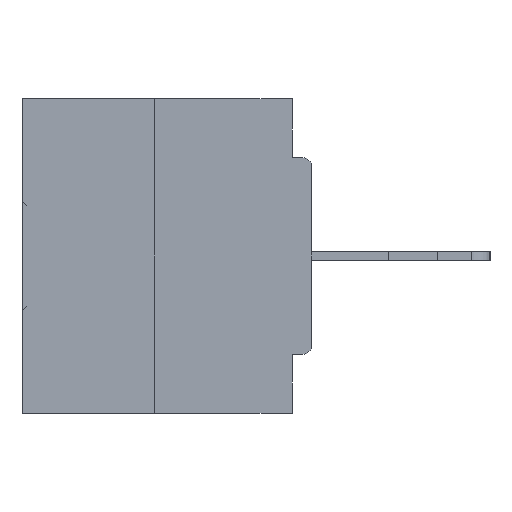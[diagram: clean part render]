
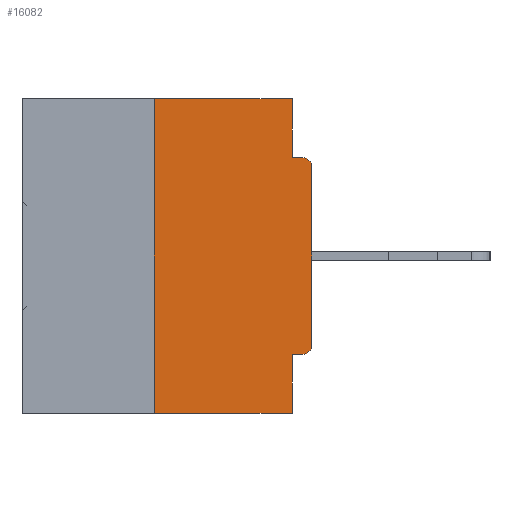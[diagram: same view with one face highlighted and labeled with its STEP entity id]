
A CAD part, left-side view. The second image highlights one B-rep face of the part: STEP entity #16082.
In plain terms, the highlighted planar face has unit normal (-1, 0, 0).
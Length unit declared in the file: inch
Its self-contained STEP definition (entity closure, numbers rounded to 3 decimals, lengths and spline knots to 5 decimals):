
#166 = CARTESIAN_POINT ( 'NONE',  ( 0., 0.031, -0.5 ) ) ;
#271 = DIRECTION ( 'NONE',  ( 0., 1., 0. ) ) ;
#1681 = DIRECTION ( 'NONE',  ( 0., 0., -1. ) ) ;
#2871 = CARTESIAN_POINT ( 'NONE',  ( 0., 0.031, -0.4065 ) ) ;
#3546 = DIRECTION ( 'NONE',  ( 0., 0., -1. ) ) ;
#4654 = CARTESIAN_POINT ( 'NONE',  ( 0., 0., -0.3915 ) ) ;
#5396 = CARTESIAN_POINT ( 'NONE',  ( 0., 0.015, -0.0935 ) ) ;
#5645 = CARTESIAN_POINT ( 'NONE',  ( 0., 0.25, -0.5 ) ) ;
#6188 = VERTEX_POINT ( 'NONE', #2871 ) ;
#6220 = CARTESIAN_POINT ( 'NONE',  ( 0., 0., -0.4065 ) ) ;
#7748 = ORIENTED_EDGE ( 'NONE', *, *, #12546, .T. ) ;
#8035 = CARTESIAN_POINT ( 'NONE',  ( 0., 0.031, -0.5 ) ) ;
#8219 = CARTESIAN_POINT ( 'NONE',  ( 0., 0., -0.0935 ) ) ;
#9398 = EDGE_LOOP ( 'NONE', ( #33979, #33507, #30368, #36195, #10634, #37885, #7748, #32452, #12230, #32280 ) ) ;
#9881 = CARTESIAN_POINT ( 'NONE',  ( 0., 0.031, 0. ) ) ;
#9919 = DIRECTION ( 'NONE',  ( -1., 0., 0. ) ) ;
#10634 = ORIENTED_EDGE ( 'NONE', *, *, #40237, .F. ) ;
#10736 = DIRECTION ( 'NONE',  ( -1., 0., 0. ) ) ;
#11632 = LINE ( 'NONE', #20674, #40457 ) ;
#12211 = EDGE_CURVE ( 'NONE', #38608, #39291, #38129, .T. ) ;
#12230 = ORIENTED_EDGE ( 'NONE', *, *, #25489, .F. ) ;
#12546 = EDGE_CURVE ( 'NONE', #26286, #21401, #11632, .T. ) ;
#14592 = FACE_OUTER_BOUND ( 'NONE', #9398, .T. ) ;
#15478 = EDGE_CURVE ( 'NONE', #6188, #39291, #18635, .T. ) ;
#16082 = ADVANCED_FACE ( 'NONE', ( #14592 ), #23435, .F. ) ;
#16759 = CARTESIAN_POINT ( 'NONE',  ( 0., 0.031, 0. ) ) ;
#17078 = CARTESIAN_POINT ( 'NONE',  ( 0., 0.015, -0.1085 ) ) ;
#17314 = LINE ( 'NONE', #26383, #34043 ) ;
#17432 = EDGE_CURVE ( 'NONE', #24392, #33461, #17314, .T. ) ;
#17445 = DIRECTION ( 'NONE',  ( 0., -1., 0. ) ) ;
#17661 = AXIS2_PLACEMENT_3D ( 'NONE', #28186, #9919, #3546 ) ;
#18257 = CARTESIAN_POINT ( 'NONE',  ( 0., 0.25, 0. ) ) ;
#18635 = LINE ( 'NONE', #166, #39279 ) ;
#18839 = DIRECTION ( 'NONE',  ( 0., 0., 1. ) ) ;
#19458 = CARTESIAN_POINT ( 'NONE',  ( 0., 0.46, -0.5 ) ) ;
#19953 = DIRECTION ( 'NONE',  ( 1., 0., 0. ) ) ;
#19972 = DIRECTION ( 'NONE',  ( 0., 0., -1. ) ) ;
#20674 = CARTESIAN_POINT ( 'NONE',  ( 0., 0., 0. ) ) ;
#21401 = VERTEX_POINT ( 'NONE', #38462 ) ;
#22126 = DIRECTION ( 'NONE',  ( 0., 0., -1. ) ) ;
#22452 = AXIS2_PLACEMENT_3D ( 'NONE', #17078, #10736, #19972 ) ;
#22699 = VECTOR ( 'NONE', #17445, 39.37008 ) ;
#23435 = PLANE ( 'NONE',  #26215 ) ;
#24304 = DIRECTION ( 'NONE',  ( 0., -1., 0. ) ) ;
#24392 = VERTEX_POINT ( 'NONE', #18257 ) ;
#24836 = VECTOR ( 'NONE', #18839, 39.37008 ) ;
#25211 = CARTESIAN_POINT ( 'NONE',  ( 0., 0.25, 0. ) ) ;
#25489 = EDGE_CURVE ( 'NONE', #27719, #30728, #40005, .T. ) ;
#26215 = AXIS2_PLACEMENT_3D ( 'NONE', #35519, #19953, #1681 ) ;
#26286 = VERTEX_POINT ( 'NONE', #4654 ) ;
#26383 = CARTESIAN_POINT ( 'NONE',  ( 0., 0.46, 0. ) ) ;
#26784 = CARTESIAN_POINT ( 'NONE',  ( 0., 0.015, -0.4065 ) ) ;
#27719 = VERTEX_POINT ( 'NONE', #34202 ) ;
#28186 = CARTESIAN_POINT ( 'NONE',  ( 0., 0.015, -0.3915 ) ) ;
#28669 = VECTOR ( 'NONE', #24304, 39.37008 ) ;
#30368 = ORIENTED_EDGE ( 'NONE', *, *, #12211, .T. ) ;
#30503 = DIRECTION ( 'NONE',  ( 0., 0., 1. ) ) ;
#30713 = VECTOR ( 'NONE', #38919, 39.37008 ) ;
#30728 = VERTEX_POINT ( 'NONE', #5396 ) ;
#31062 = LINE ( 'NONE', #6220, #37327 ) ;
#31638 = VERTEX_POINT ( 'NONE', #26784 ) ;
#32280 = ORIENTED_EDGE ( 'NONE', *, *, #39494, .F. ) ;
#32452 = ORIENTED_EDGE ( 'NONE', *, *, #33124, .T. ) ;
#33124 = EDGE_CURVE ( 'NONE', #21401, #30728, #34238, .T. ) ;
#33461 = VERTEX_POINT ( 'NONE', #9881 ) ;
#33507 = ORIENTED_EDGE ( 'NONE', *, *, #39416, .F. ) ;
#33979 = ORIENTED_EDGE ( 'NONE', *, *, #17432, .F. ) ;
#34043 = VECTOR ( 'NONE', #38871, 39.37008 ) ;
#34202 = CARTESIAN_POINT ( 'NONE',  ( 0., 0.031, -0.0935 ) ) ;
#34238 = CIRCLE ( 'NONE', #22452, 0.015 ) ;
#35519 = CARTESIAN_POINT ( 'NONE',  ( 0., 0.46, 0. ) ) ;
#36195 = ORIENTED_EDGE ( 'NONE', *, *, #15478, .F. ) ;
#37303 = LINE ( 'NONE', #25211, #24836 ) ;
#37327 = VECTOR ( 'NONE', #271, 39.37008 ) ;
#37885 = ORIENTED_EDGE ( 'NONE', *, *, #40295, .T. ) ;
#38129 = LINE ( 'NONE', #19458, #28669 ) ;
#38462 = CARTESIAN_POINT ( 'NONE',  ( 0., 0., -0.1085 ) ) ;
#38608 = VERTEX_POINT ( 'NONE', #5645 ) ;
#38720 = LINE ( 'NONE', #16759, #30713 ) ;
#38871 = DIRECTION ( 'NONE',  ( 0., -1., 0. ) ) ;
#38919 = DIRECTION ( 'NONE',  ( 0., 0., -1. ) ) ;
#39279 = VECTOR ( 'NONE', #22126, 39.37008 ) ;
#39291 = VERTEX_POINT ( 'NONE', #8035 ) ;
#39416 = EDGE_CURVE ( 'NONE', #38608, #24392, #37303, .T. ) ;
#39494 = EDGE_CURVE ( 'NONE', #33461, #27719, #38720, .T. ) ;
#39916 = CIRCLE ( 'NONE', #17661, 0.015 ) ;
#40005 = LINE ( 'NONE', #8219, #22699 ) ;
#40237 = EDGE_CURVE ( 'NONE', #31638, #6188, #31062, .T. ) ;
#40295 = EDGE_CURVE ( 'NONE', #31638, #26286, #39916, .T. ) ;
#40457 = VECTOR ( 'NONE', #30503, 39.37008 ) ;
